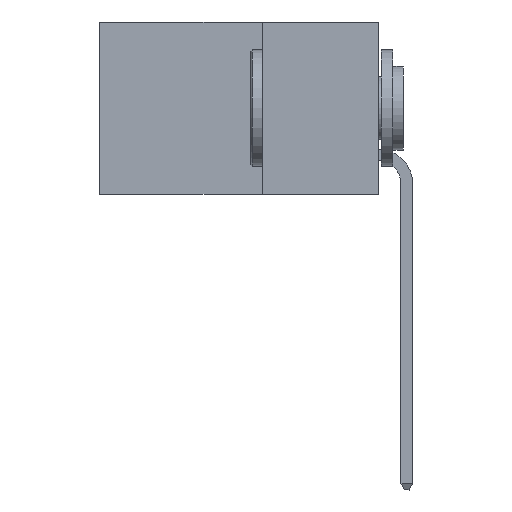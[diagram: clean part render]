
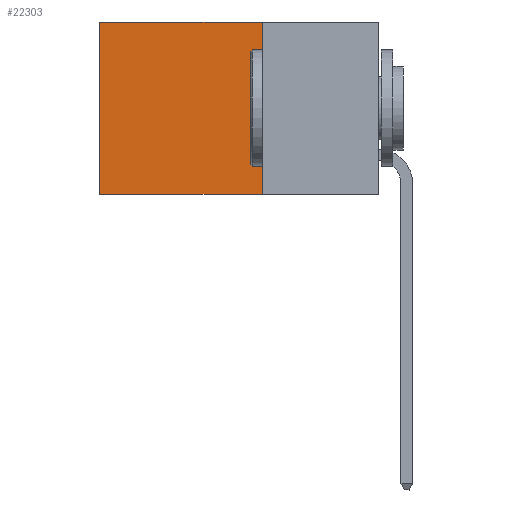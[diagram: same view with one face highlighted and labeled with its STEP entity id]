
A CAD part, left-side view. The second image highlights one B-rep face of the part: STEP entity #22303.
In plain terms, the highlighted planar face has unit normal (-1, 0, 0).
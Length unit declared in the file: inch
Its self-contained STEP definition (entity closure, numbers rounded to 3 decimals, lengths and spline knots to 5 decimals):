
#29 = EDGE_CURVE ( 'NONE', #19579, #13699, #15337, .T. ) ;
#1913 = LINE ( 'NONE', #11237, #4800 ) ;
#2638 = FACE_OUTER_BOUND ( 'NONE', #3306, .T. ) ;
#3306 = EDGE_LOOP ( 'NONE', ( #22045, #6844, #22947, #19708 ) ) ;
#3823 = AXIS2_PLACEMENT_3D ( 'NONE', #21081, #4345, #4584 ) ;
#4206 = DIRECTION ( 'NONE',  ( 0., 1., 0. ) ) ;
#4345 = DIRECTION ( 'NONE',  ( 1., 0., 0. ) ) ;
#4584 = DIRECTION ( 'NONE',  ( 0., 0., -1. ) ) ;
#4800 = VECTOR ( 'NONE', #9425, 39.37008 ) ;
#6730 = DIRECTION ( 'NONE',  ( 0., 0., -1. ) ) ;
#6844 = ORIENTED_EDGE ( 'NONE', *, *, #17469, .F. ) ;
#7369 = DIRECTION ( 'NONE',  ( 0., 0., -1. ) ) ;
#9170 = LINE ( 'NONE', #13145, #23032 ) ;
#9425 = DIRECTION ( 'NONE',  ( 0., 1., 0. ) ) ;
#9477 = CARTESIAN_POINT ( 'NONE',  ( 0.2615, 0.25, -0.37 ) ) ;
#11237 = CARTESIAN_POINT ( 'NONE',  ( 0.2615, 0.25, -0.37 ) ) ;
#11461 = CARTESIAN_POINT ( 'NONE',  ( 0.2615, 0.6, -0.37 ) ) ;
#11924 = CARTESIAN_POINT ( 'NONE',  ( 0.2615, 0.25, 0. ) ) ;
#12258 = LINE ( 'NONE', #23128, #15249 ) ;
#13145 = CARTESIAN_POINT ( 'NONE',  ( 0.2615, 0.25, -0.37 ) ) ;
#13642 = PLANE ( 'NONE',  #3823 ) ;
#13699 = VERTEX_POINT ( 'NONE', #23987 ) ;
#14592 = VERTEX_POINT ( 'NONE', #11461 ) ;
#15249 = VECTOR ( 'NONE', #6730, 39.37008 ) ;
#15337 = LINE ( 'NONE', #20344, #21115 ) ;
#17469 = EDGE_CURVE ( 'NONE', #21061, #14592, #1913, .T. ) ;
#17914 = EDGE_CURVE ( 'NONE', #13699, #14592, #12258, .T. ) ;
#18899 = EDGE_CURVE ( 'NONE', #19579, #21061, #9170, .T. ) ;
#19579 = VERTEX_POINT ( 'NONE', #11924 ) ;
#19708 = ORIENTED_EDGE ( 'NONE', *, *, #29, .T. ) ;
#20344 = CARTESIAN_POINT ( 'NONE',  ( 0.2615, 0.25, 0. ) ) ;
#21061 = VERTEX_POINT ( 'NONE', #9477 ) ;
#21081 = CARTESIAN_POINT ( 'NONE',  ( 0.2615, 0.25, -0.37 ) ) ;
#21115 = VECTOR ( 'NONE', #4206, 39.37008 ) ;
#22045 = ORIENTED_EDGE ( 'NONE', *, *, #17914, .T. ) ;
#22303 = ADVANCED_FACE ( 'NONE', ( #2638 ), #13642, .F. ) ;
#22947 = ORIENTED_EDGE ( 'NONE', *, *, #18899, .F. ) ;
#23032 = VECTOR ( 'NONE', #7369, 39.37008 ) ;
#23128 = CARTESIAN_POINT ( 'NONE',  ( 0.2615, 0.6, -0.37 ) ) ;
#23987 = CARTESIAN_POINT ( 'NONE',  ( 0.2615, 0.6, 0. ) ) ;
